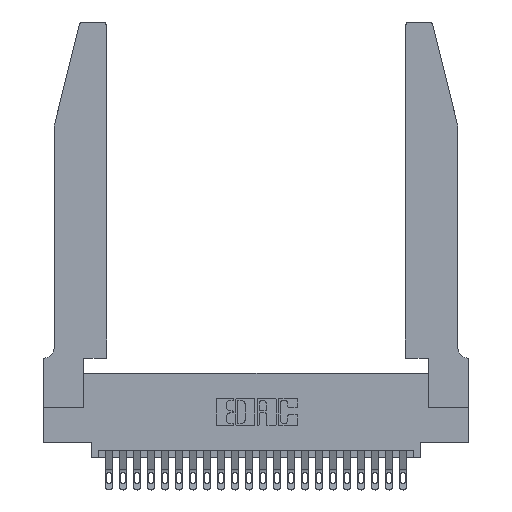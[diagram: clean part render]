
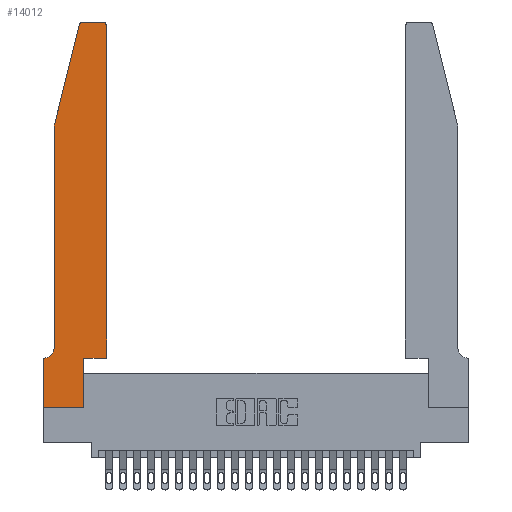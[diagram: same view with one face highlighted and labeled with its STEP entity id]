
A CAD part, top view. The second image highlights one B-rep face of the part: STEP entity #14012.
In plain terms, the highlighted planar face has unit normal (0, 0, 1).
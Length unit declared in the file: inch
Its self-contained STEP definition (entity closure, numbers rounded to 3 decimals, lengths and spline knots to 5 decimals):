
#200 = EDGE_CURVE ( 'NONE', #15315, #6952, #9385, .T. ) ;
#421 = EDGE_CURVE ( 'NONE', #12389, #1687, #12795, .T. ) ;
#635 = DIRECTION ( 'NONE',  ( 0., -1., 0. ) ) ;
#988 = DIRECTION ( 'NONE',  ( 1., 0., 0. ) ) ;
#1102 = LINE ( 'NONE', #8490, #14538 ) ;
#1352 = CARTESIAN_POINT ( 'NONE',  ( 0.0755, 2., 0.37 ) ) ;
#1687 = VERTEX_POINT ( 'NONE', #2974 ) ;
#1783 = CARTESIAN_POINT ( 'NONE',  ( 0.2865, 0.35, 0.37 ) ) ;
#1910 = DIRECTION ( 'NONE',  ( -0.239, -0.971, 0. ) ) ;
#2265 = AXIS2_PLACEMENT_3D ( 'NONE', #23857, #10304, #19997 ) ;
#2857 = DIRECTION ( 'NONE',  ( 0., 0., 1. ) ) ;
#2974 = CARTESIAN_POINT ( 'NONE',  ( 0.4205, 2.75, 0.37 ) ) ;
#3257 = VERTEX_POINT ( 'NONE', #8421 ) ;
#3298 = CARTESIAN_POINT ( 'NONE',  ( 0.0055, 0.35, 0.37 ) ) ;
#3311 = DIRECTION ( 'NONE',  ( 1., 0., 0. ) ) ;
#3391 = DIRECTION ( 'NONE',  ( 0., -1., 0. ) ) ;
#3531 = LINE ( 'NONE', #1352, #5615 ) ;
#3810 = CARTESIAN_POINT ( 'NONE',  ( 0.0755, 2., 0.37 ) ) ;
#5371 = ORIENTED_EDGE ( 'NONE', *, *, #16717, .T. ) ;
#5416 = VERTEX_POINT ( 'NONE', #9815 ) ;
#5615 = VECTOR ( 'NONE', #3391, 39.37008 ) ;
#5660 = DIRECTION ( 'NONE',  ( 0., 0., -1. ) ) ;
#5729 = VECTOR ( 'NONE', #1910, 39.37008 ) ;
#5735 = CARTESIAN_POINT ( 'NONE',  ( 0.25487, 2.72718, 0.37 ) ) ;
#5849 = VECTOR ( 'NONE', #13164, 39.37008 ) ;
#6133 = CARTESIAN_POINT ( 'NONE',  ( 0., 0., 0.37 ) ) ;
#6308 = PLANE ( 'NONE',  #12521 ) ;
#6327 = CARTESIAN_POINT ( 'NONE',  ( 0.2865, 0., 0.37 ) ) ;
#6565 = DIRECTION ( 'NONE',  ( 0., 1., 0. ) ) ;
#6676 = ORIENTED_EDGE ( 'NONE', *, *, #10512, .T. ) ;
#6952 = VERTEX_POINT ( 'NONE', #6133 ) ;
#7029 = EDGE_CURVE ( 'NONE', #3257, #15110, #9403, .T. ) ;
#7267 = CARTESIAN_POINT ( 'NONE',  ( 0.4505, 0.35, 0.37 ) ) ;
#7278 = EDGE_CURVE ( 'NONE', #17000, #15315, #20440, .T. ) ;
#7407 = VECTOR ( 'NONE', #7810, 39.37008 ) ;
#7810 = DIRECTION ( 'NONE',  ( 1., 0., 0. ) ) ;
#8421 = CARTESIAN_POINT ( 'NONE',  ( 0.284, 2.75, 0.37 ) ) ;
#8490 = CARTESIAN_POINT ( 'NONE',  ( 0.4505, 0.35, 0.37 ) ) ;
#8594 = CARTESIAN_POINT ( 'NONE',  ( 0., 0.35, 0.37 ) ) ;
#8711 = CARTESIAN_POINT ( 'NONE',  ( 0.4505, 2.72, 0.37 ) ) ;
#8767 = LINE ( 'NONE', #16578, #11519 ) ;
#8786 = VECTOR ( 'NONE', #635, 39.37008 ) ;
#9297 = EDGE_CURVE ( 'NONE', #1687, #3257, #8767, .T. ) ;
#9385 = LINE ( 'NONE', #23928, #8786 ) ;
#9403 = CIRCLE ( 'NONE', #2265, 0.03 ) ;
#9479 = ORIENTED_EDGE ( 'NONE', *, *, #9297, .T. ) ;
#9633 = AXIS2_PLACEMENT_3D ( 'NONE', #13628, #5660, #13544 ) ;
#9815 = CARTESIAN_POINT ( 'NONE',  ( 0.4505, 0.35, 0.37 ) ) ;
#10002 = VECTOR ( 'NONE', #11176, 39.37008 ) ;
#10102 = EDGE_CURVE ( 'NONE', #12125, #17000, #20963, .T. ) ;
#10225 = LINE ( 'NONE', #7267, #20645 ) ;
#10304 = DIRECTION ( 'NONE',  ( 0., 0., 1. ) ) ;
#10512 = EDGE_CURVE ( 'NONE', #19477, #5416, #10225, .T. ) ;
#10947 = CARTESIAN_POINT ( 'NONE',  ( 0.0755, 2., 0.37 ) ) ;
#11057 = LINE ( 'NONE', #13012, #5849 ) ;
#11176 = DIRECTION ( 'NONE',  ( -1., 0., 0. ) ) ;
#11309 = ORIENTED_EDGE ( 'NONE', *, *, #200, .T. ) ;
#11519 = VECTOR ( 'NONE', #12725, 39.37008 ) ;
#11531 = ORIENTED_EDGE ( 'NONE', *, *, #10102, .T. ) ;
#11746 = ORIENTED_EDGE ( 'NONE', *, *, #21081, .T. ) ;
#11941 = VERTEX_POINT ( 'NONE', #3810 ) ;
#12072 = ORIENTED_EDGE ( 'NONE', *, *, #13166, .T. ) ;
#12125 = VERTEX_POINT ( 'NONE', #17947 ) ;
#12389 = VERTEX_POINT ( 'NONE', #8711 ) ;
#12516 = CARTESIAN_POINT ( 'NONE',  ( 0., 0.35, 0.37 ) ) ;
#12521 = AXIS2_PLACEMENT_3D ( 'NONE', #8594, #2857, #988 ) ;
#12725 = DIRECTION ( 'NONE',  ( -1., 0., 0. ) ) ;
#12795 = CIRCLE ( 'NONE', #13925, 0.03 ) ;
#13012 = CARTESIAN_POINT ( 'NONE',  ( 0.2865, 0.35, 0.37 ) ) ;
#13067 = ORIENTED_EDGE ( 'NONE', *, *, #7029, .T. ) ;
#13164 = DIRECTION ( 'NONE',  ( 0., 1., 0. ) ) ;
#13166 = EDGE_CURVE ( 'NONE', #6952, #23955, #19943, .T. ) ;
#13455 = ORIENTED_EDGE ( 'NONE', *, *, #18613, .T. ) ;
#13523 = ORIENTED_EDGE ( 'NONE', *, *, #421, .T. ) ;
#13544 = DIRECTION ( 'NONE',  ( -1., 0., 0. ) ) ;
#13628 = CARTESIAN_POINT ( 'NONE',  ( 0.0055, 0.42, 0.37 ) ) ;
#13925 = AXIS2_PLACEMENT_3D ( 'NONE', #16923, #24724, #17085 ) ;
#14012 = ADVANCED_FACE ( 'NONE', ( #16552 ), #6308, .T. ) ;
#14538 = VECTOR ( 'NONE', #6565, 39.37008 ) ;
#15110 = VERTEX_POINT ( 'NONE', #5735 ) ;
#15315 = VERTEX_POINT ( 'NONE', #12516 ) ;
#16552 = FACE_OUTER_BOUND ( 'NONE', #23981, .T. ) ;
#16578 = CARTESIAN_POINT ( 'NONE',  ( 0.2605, 2.75, 0.37 ) ) ;
#16717 = EDGE_CURVE ( 'NONE', #11941, #12125, #3531, .T. ) ;
#16923 = CARTESIAN_POINT ( 'NONE',  ( 0.4205, 2.72, 0.37 ) ) ;
#17000 = VERTEX_POINT ( 'NONE', #3298 ) ;
#17085 = DIRECTION ( 'NONE',  ( 1., 0., 0. ) ) ;
#17368 = LINE ( 'NONE', #10947, #5729 ) ;
#17435 = EDGE_CURVE ( 'NONE', #5416, #12389, #1102, .T. ) ;
#17853 = ORIENTED_EDGE ( 'NONE', *, *, #7278, .T. ) ;
#17947 = CARTESIAN_POINT ( 'NONE',  ( 0.0755, 0.42, 0.37 ) ) ;
#18613 = EDGE_CURVE ( 'NONE', #23955, #19477, #11057, .T. ) ;
#19477 = VERTEX_POINT ( 'NONE', #1783 ) ;
#19943 = LINE ( 'NONE', #23341, #7407 ) ;
#19997 = DIRECTION ( 'NONE',  ( 1., 0., 0. ) ) ;
#20440 = LINE ( 'NONE', #22771, #10002 ) ;
#20645 = VECTOR ( 'NONE', #3311, 39.37008 ) ;
#20963 = CIRCLE ( 'NONE', #9633, 0.07 ) ;
#21081 = EDGE_CURVE ( 'NONE', #15110, #11941, #17368, .T. ) ;
#22771 = CARTESIAN_POINT ( 'NONE',  ( 0.0755, 0.35, 0.37 ) ) ;
#23281 = ORIENTED_EDGE ( 'NONE', *, *, #17435, .T. ) ;
#23341 = CARTESIAN_POINT ( 'NONE',  ( 0., 0., 0.37 ) ) ;
#23857 = CARTESIAN_POINT ( 'NONE',  ( 0.284, 2.72, 0.37 ) ) ;
#23928 = CARTESIAN_POINT ( 'NONE',  ( 0., 0., 0.37 ) ) ;
#23955 = VERTEX_POINT ( 'NONE', #6327 ) ;
#23981 = EDGE_LOOP ( 'NONE', ( #9479, #13067, #11746, #5371, #11531, #17853, #11309, #12072, #13455, #6676, #23281, #13523 ) ) ;
#24724 = DIRECTION ( 'NONE',  ( 0., 0., 1. ) ) ;
